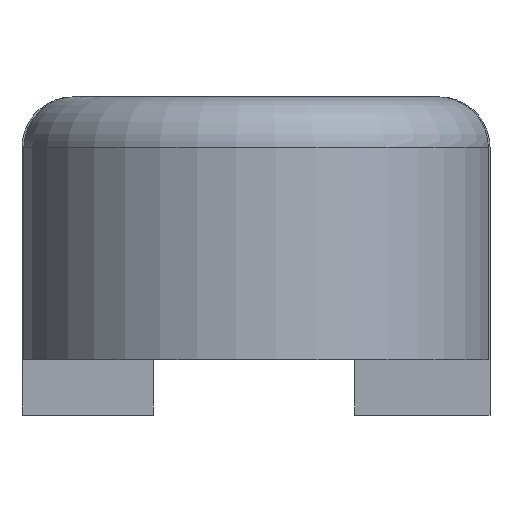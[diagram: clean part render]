
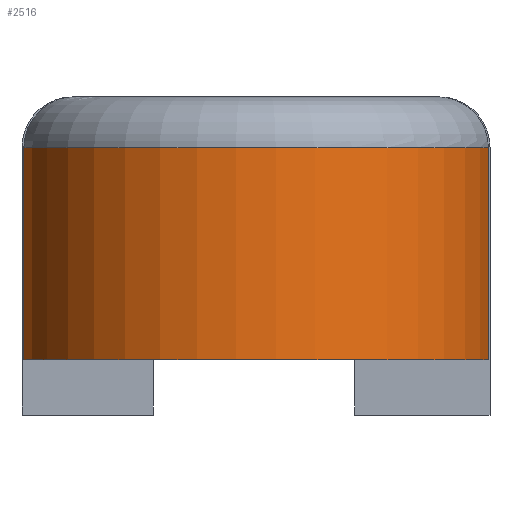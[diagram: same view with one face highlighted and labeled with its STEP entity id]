
A CAD part, front view. The second image highlights one B-rep face of the part: STEP entity #2516.
In plain terms, the highlighted cylindrical face has radius 18.556 mm (diameter 37.112 mm), a partial arc.
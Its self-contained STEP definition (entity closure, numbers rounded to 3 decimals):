
#32 = PLANE('',#33);
#33 = AXIS2_PLACEMENT_3D('',#34,#35,#36);
#34 = CARTESIAN_POINT('',(76.839,42.673,-31.75));
#35 = DIRECTION('',(0.,-1.,0.));
#36 = DIRECTION('',(-1.,0.,0.));
#110 = VERTEX_POINT('',#111);
#111 = CARTESIAN_POINT('',(39.267,42.673,0.));
#135 = EDGE_CURVE('',#136,#110,#138,.T.);
#136 = VERTEX_POINT('',#137);
#137 = CARTESIAN_POINT('',(39.267,42.673,16.8));
#138 = SURFACE_CURVE('',#139,(#143,#149),.PCURVE_S1.);
#139 = LINE('',#140,#141);
#140 = CARTESIAN_POINT('',(39.267,42.673,0.));
#141 = VECTOR('',#142,1.);
#142 = DIRECTION('',(0.,0.,-1.));
#143 = PCURVE('',#32,#144);
#144 = DEFINITIONAL_REPRESENTATION('',(#145),#148);
#145 = B_SPLINE_CURVE_WITH_KNOTS('',1,(#146,#147),.UNSPECIFIED.,.F.,.F.,
  (2,2),(-20.8,0.),.PIECEWISE_BEZIER_KNOTS.);
#146 = CARTESIAN_POINT('',(37.572,-52.55));
#147 = CARTESIAN_POINT('',(37.572,-31.75));
#148 = ( GEOMETRIC_REPRESENTATION_CONTEXT(2) 
PARAMETRIC_REPRESENTATION_CONTEXT() REPRESENTATION_CONTEXT('2D SPACE',''
  ) );
#149 = PCURVE('',#150,#155);
#150 = CYLINDRICAL_SURFACE('',#151,18.556);
#151 = AXIS2_PLACEMENT_3D('',#152,#153,#154);
#152 = CARTESIAN_POINT('',(57.665,45.086,0.));
#153 = DIRECTION('',(0.,0.,-1.));
#154 = DIRECTION('',(1.,0.,0.));
#155 = DEFINITIONAL_REPRESENTATION('',(#156),#159);
#156 = B_SPLINE_CURVE_WITH_KNOTS('',1,(#157,#158),.UNSPECIFIED.,.F.,.F.,
  (2,2),(-20.8,0.),.PIECEWISE_BEZIER_KNOTS.);
#157 = CARTESIAN_POINT('',(-3.272,-20.8));
#158 = CARTESIAN_POINT('',(-3.272,0.));
#159 = ( GEOMETRIC_REPRESENTATION_CONTEXT(2) 
PARAMETRIC_REPRESENTATION_CONTEXT() REPRESENTATION_CONTEXT('2D SPACE',''
  ) );
#373 = TOROIDAL_SURFACE('',#374,14.556,4.);
#374 = AXIS2_PLACEMENT_3D('',#375,#376,#377);
#375 = CARTESIAN_POINT('',(57.665,45.086,16.8));
#376 = DIRECTION('',(0.,0.,1.));
#377 = DIRECTION('',(-0.992,-0.13,0.));
#510 = VERTEX_POINT('',#511);
#511 = CARTESIAN_POINT('',(76.063,42.673,16.8));
#826 = EDGE_CURVE('',#510,#827,#829,.T.);
#827 = VERTEX_POINT('',#828);
#828 = CARTESIAN_POINT('',(76.063,42.673,0.));
#829 = SURFACE_CURVE('',#830,(#834,#840),.PCURVE_S1.);
#830 = LINE('',#831,#832);
#831 = CARTESIAN_POINT('',(76.063,42.673,0.));
#832 = VECTOR('',#833,1.);
#833 = DIRECTION('',(0.,0.,-1.));
#834 = PCURVE('',#32,#835);
#835 = DEFINITIONAL_REPRESENTATION('',(#836),#839);
#836 = B_SPLINE_CURVE_WITH_KNOTS('',1,(#837,#838),.UNSPECIFIED.,.F.,.F.,
  (2,2),(-20.8,0.),.PIECEWISE_BEZIER_KNOTS.);
#837 = CARTESIAN_POINT('',(0.776,-52.55));
#838 = CARTESIAN_POINT('',(0.776,-31.75));
#839 = ( GEOMETRIC_REPRESENTATION_CONTEXT(2) 
PARAMETRIC_REPRESENTATION_CONTEXT() REPRESENTATION_CONTEXT('2D SPACE',''
  ) );
#840 = PCURVE('',#150,#841);
#841 = DEFINITIONAL_REPRESENTATION('',(#842),#845);
#842 = B_SPLINE_CURVE_WITH_KNOTS('',1,(#843,#844),.UNSPECIFIED.,.F.,.F.,
  (2,2),(-20.8,0.),.PIECEWISE_BEZIER_KNOTS.);
#843 = CARTESIAN_POINT('',(-6.153,-20.8));
#844 = CARTESIAN_POINT('',(-6.153,0.));
#845 = ( GEOMETRIC_REPRESENTATION_CONTEXT(2) 
PARAMETRIC_REPRESENTATION_CONTEXT() REPRESENTATION_CONTEXT('2D SPACE',''
  ) );
#2516 = ADVANCED_FACE('',(#2517),#150,.T.);
#2517 = FACE_BOUND('',#2518,.F.);
#2518 = EDGE_LOOP('',(#2519,#2520,#2551,#2552));
#2519 = ORIENTED_EDGE('',*,*,#826,.T.);
#2520 = ORIENTED_EDGE('',*,*,#2521,.F.);
#2521 = EDGE_CURVE('',#110,#827,#2522,.T.);
#2522 = SURFACE_CURVE('',#2523,(#2528,#2535),.PCURVE_S1.);
#2523 = CIRCLE('',#2524,18.556);
#2524 = AXIS2_PLACEMENT_3D('',#2525,#2526,#2527);
#2525 = CARTESIAN_POINT('',(57.665,45.086,0.));
#2526 = DIRECTION('',(0.,0.,1.));
#2527 = DIRECTION('',(1.,0.,0.));
#2528 = PCURVE('',#150,#2529);
#2529 = DEFINITIONAL_REPRESENTATION('',(#2530),#2534);
#2530 = LINE('',#2531,#2532);
#2531 = CARTESIAN_POINT('',(0.,0.));
#2532 = VECTOR('',#2533,1.);
#2533 = DIRECTION('',(-1.,0.));
#2534 = ( GEOMETRIC_REPRESENTATION_CONTEXT(2) 
PARAMETRIC_REPRESENTATION_CONTEXT() REPRESENTATION_CONTEXT('2D SPACE',''
  ) );
#2535 = PCURVE('',#2536,#2541);
#2536 = PLANE('',#2537);
#2537 = AXIS2_PLACEMENT_3D('',#2538,#2539,#2540);
#2538 = CARTESIAN_POINT('',(39.165,43.648,0.));
#2539 = DIRECTION('',(0.,0.,-1.));
#2540 = DIRECTION('',(-1.,0.,0.));
#2541 = DEFINITIONAL_REPRESENTATION('',(#2542),#2550);
#2542 = ( BOUNDED_CURVE() B_SPLINE_CURVE(2,(#2543,#2544,#2545,#2546,
#2547,#2548,#2549),.UNSPECIFIED.,.T.,.F.) B_SPLINE_CURVE_WITH_KNOTS((1,2
    ,2,2,2,1),(-2.094,0.,2.094,4.189,
6.283,8.378),.UNSPECIFIED.) CURVE() 
GEOMETRIC_REPRESENTATION_ITEM() RATIONAL_B_SPLINE_CURVE((1.,0.5,1.,0.5,
1.,0.5,1.)) REPRESENTATION_ITEM('') );
#2543 = CARTESIAN_POINT('',(-37.056,1.438));
#2544 = CARTESIAN_POINT('',(-37.056,33.578));
#2545 = CARTESIAN_POINT('',(-9.222,17.508));
#2546 = CARTESIAN_POINT('',(18.612,1.438));
#2547 = CARTESIAN_POINT('',(-9.222,-14.632));
#2548 = CARTESIAN_POINT('',(-37.056,-30.702));
#2549 = CARTESIAN_POINT('',(-37.056,1.438));
#2550 = ( GEOMETRIC_REPRESENTATION_CONTEXT(2) 
PARAMETRIC_REPRESENTATION_CONTEXT() REPRESENTATION_CONTEXT('2D SPACE',''
  ) );
#2551 = ORIENTED_EDGE('',*,*,#135,.F.);
#2552 = ORIENTED_EDGE('',*,*,#2553,.T.);
#2553 = EDGE_CURVE('',#136,#510,#2554,.T.);
#2554 = SURFACE_CURVE('',#2555,(#2560,#2567),.PCURVE_S1.);
#2555 = CIRCLE('',#2556,18.556);
#2556 = AXIS2_PLACEMENT_3D('',#2557,#2558,#2559);
#2557 = CARTESIAN_POINT('',(57.665,45.086,16.8));
#2558 = DIRECTION('',(0.,0.,1.));
#2559 = DIRECTION('',(-0.992,-0.13,0.));
#2560 = PCURVE('',#150,#2561);
#2561 = DEFINITIONAL_REPRESENTATION('',(#2562),#2566);
#2562 = LINE('',#2563,#2564);
#2563 = CARTESIAN_POINT('',(-3.272,-16.8));
#2564 = VECTOR('',#2565,1.);
#2565 = DIRECTION('',(-1.,0.));
#2566 = ( GEOMETRIC_REPRESENTATION_CONTEXT(2) 
PARAMETRIC_REPRESENTATION_CONTEXT() REPRESENTATION_CONTEXT('2D SPACE',''
  ) );
#2567 = PCURVE('',#373,#2568);
#2568 = DEFINITIONAL_REPRESENTATION('',(#2569),#2573);
#2569 = LINE('',#2570,#2571);
#2570 = CARTESIAN_POINT('',(0.,0.));
#2571 = VECTOR('',#2572,1.);
#2572 = DIRECTION('',(1.,0.));
#2573 = ( GEOMETRIC_REPRESENTATION_CONTEXT(2) 
PARAMETRIC_REPRESENTATION_CONTEXT() REPRESENTATION_CONTEXT('2D SPACE',''
  ) );
